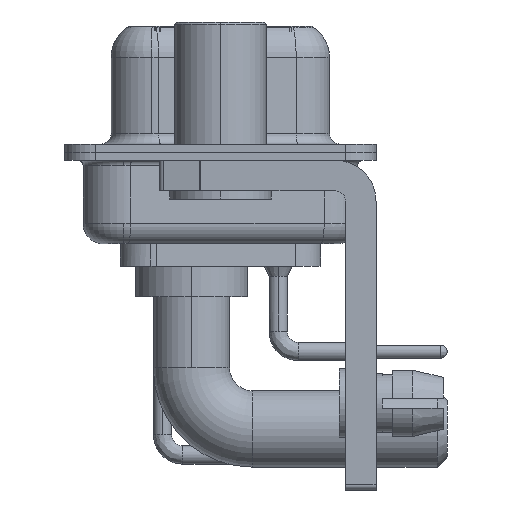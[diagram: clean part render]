
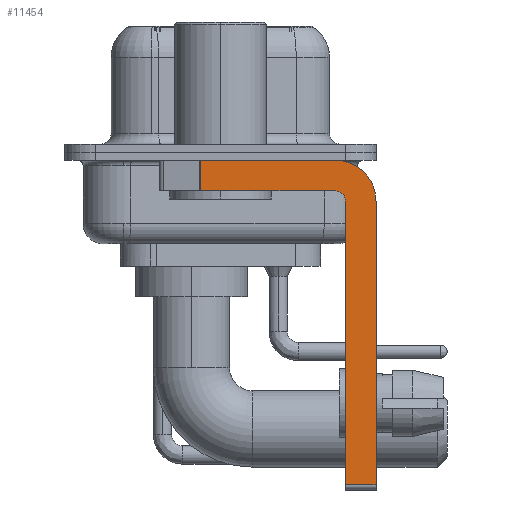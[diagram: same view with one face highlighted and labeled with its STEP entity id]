
A CAD part, left-side view. The second image highlights one B-rep face of the part: STEP entity #11454.
In plain terms, the highlighted planar face has unit normal (-1, 0, 0).
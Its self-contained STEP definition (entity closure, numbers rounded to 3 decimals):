
#1162 = DIRECTION ( 'NONE',  ( 0., 0., -1. ) ) ;
#2104 = VECTOR ( 'NONE', #4089, 1000. ) ;
#2225 = AXIS2_PLACEMENT_3D ( 'NONE', #18593, #27912, #32994 ) ;
#2735 = DIRECTION ( 'NONE',  ( 0., -1., 0. ) ) ;
#3118 = EDGE_LOOP ( 'NONE', ( #25243, #11658, #6169, #10209, #12812, #8840, #5963, #27214 ) ) ;
#4089 = DIRECTION ( 'NONE',  ( 0., 0., 1. ) ) ;
#4262 = CARTESIAN_POINT ( 'NONE',  ( -2.9, -6.15, -16.6 ) ) ;
#4948 = LINE ( 'NONE', #30495, #33307 ) ;
#5680 = CARTESIAN_POINT ( 'NONE',  ( -2.9, -6.15, -16.35 ) ) ;
#5963 = ORIENTED_EDGE ( 'NONE', *, *, #25046, .F. ) ;
#6169 = ORIENTED_EDGE ( 'NONE', *, *, #10638, .F. ) ;
#6309 = LINE ( 'NONE', #4262, #2104 ) ;
#6422 = CARTESIAN_POINT ( 'NONE',  ( -2.9, -5.65, -0.4 ) ) ;
#8209 = EDGE_CURVE ( 'NONE', #29471, #16272, #23534, .T. ) ;
#8766 = DIRECTION ( 'NONE',  ( 0., 1., 0. ) ) ;
#8840 = ORIENTED_EDGE ( 'NONE', *, *, #23420, .T. ) ;
#8956 = CARTESIAN_POINT ( 'NONE',  ( -2.9, 0.978, -1.9 ) ) ;
#9490 = CARTESIAN_POINT ( 'NONE',  ( -2.9, -5.65, -1.9 ) ) ;
#10067 = CIRCLE ( 'NONE', #13868, 2. ) ;
#10209 = ORIENTED_EDGE ( 'NONE', *, *, #29334, .F. ) ;
#10638 = EDGE_CURVE ( 'NONE', #16026, #17993, #26530, .T. ) ;
#10741 = VERTEX_POINT ( 'NONE', #32449 ) ;
#11454 = ADVANCED_FACE ( 'NONE', ( #15449 ), #25781, .F. ) ;
#11658 = ORIENTED_EDGE ( 'NONE', *, *, #25609, .T. ) ;
#12203 = DIRECTION ( 'NONE',  ( 0., 0., -1. ) ) ;
#12812 = ORIENTED_EDGE ( 'NONE', *, *, #27222, .F. ) ;
#13102 = DIRECTION ( 'NONE',  ( 1., 0., 0. ) ) ;
#13689 = CARTESIAN_POINT ( 'NONE',  ( -2.9, 0.978, -0.4 ) ) ;
#13868 = AXIS2_PLACEMENT_3D ( 'NONE', #29997, #22898, #30502 ) ;
#14150 = EDGE_CURVE ( 'NONE', #16272, #15991, #10067, .T. ) ;
#15449 = FACE_OUTER_BOUND ( 'NONE', #3118, .T. ) ;
#15776 = DIRECTION ( 'NONE',  ( 0., 0., -1. ) ) ;
#15991 = VERTEX_POINT ( 'NONE', #17605 ) ;
#16026 = VERTEX_POINT ( 'NONE', #9490 ) ;
#16272 = VERTEX_POINT ( 'NONE', #6422 ) ;
#16274 = CIRCLE ( 'NONE', #2225, 0.5 ) ;
#17193 = VERTEX_POINT ( 'NONE', #5680 ) ;
#17605 = CARTESIAN_POINT ( 'NONE',  ( -2.9, -7.65, -2.4 ) ) ;
#17993 = VERTEX_POINT ( 'NONE', #8956 ) ;
#18593 = CARTESIAN_POINT ( 'NONE',  ( -2.9, -5.65, -2.4 ) ) ;
#19361 = VECTOR ( 'NONE', #12203, 1000. ) ;
#20318 = DIRECTION ( 'NONE',  ( 0., -1., 0. ) ) ;
#20493 = CARTESIAN_POINT ( 'NONE',  ( -2.9, 3., -0.4 ) ) ;
#22898 = DIRECTION ( 'NONE',  ( 1., 0., 0. ) ) ;
#23420 = EDGE_CURVE ( 'NONE', #17193, #10741, #4948, .T. ) ;
#23534 = LINE ( 'NONE', #20493, #24619 ) ;
#24166 = CARTESIAN_POINT ( 'NONE',  ( -2.9, -5.65, -1.9 ) ) ;
#24619 = VECTOR ( 'NONE', #20318, 1000. ) ;
#24796 = VECTOR ( 'NONE', #1162, 1000. ) ;
#25046 = EDGE_CURVE ( 'NONE', #15991, #10741, #28970, .T. ) ;
#25243 = ORIENTED_EDGE ( 'NONE', *, *, #8209, .F. ) ;
#25609 = EDGE_CURVE ( 'NONE', #29471, #17993, #29602, .T. ) ;
#25781 = PLANE ( 'NONE',  #31094 ) ;
#26530 = LINE ( 'NONE', #24166, #31755 ) ;
#27214 = ORIENTED_EDGE ( 'NONE', *, *, #14150, .F. ) ;
#27222 = EDGE_CURVE ( 'NONE', #17193, #33394, #6309, .T. ) ;
#27595 = CARTESIAN_POINT ( 'NONE',  ( -2.9, -7.65, -2.4 ) ) ;
#27724 = CARTESIAN_POINT ( 'NONE',  ( -2.9, 0.978, -1.9 ) ) ;
#27912 = DIRECTION ( 'NONE',  ( -1., 0., 0. ) ) ;
#28495 = CARTESIAN_POINT ( 'NONE',  ( -2.9, -5.65, -2.4 ) ) ;
#28970 = LINE ( 'NONE', #27595, #19361 ) ;
#29334 = EDGE_CURVE ( 'NONE', #33394, #16026, #16274, .T. ) ;
#29471 = VERTEX_POINT ( 'NONE', #13689 ) ;
#29602 = LINE ( 'NONE', #27724, #24796 ) ;
#29997 = CARTESIAN_POINT ( 'NONE',  ( -2.9, -5.65, -2.4 ) ) ;
#30495 = CARTESIAN_POINT ( 'NONE',  ( -2.9, -5.65, -16.35 ) ) ;
#30502 = DIRECTION ( 'NONE',  ( 0., 0., -1. ) ) ;
#31094 = AXIS2_PLACEMENT_3D ( 'NONE', #28495, #13102, #15776 ) ;
#31755 = VECTOR ( 'NONE', #8766, 1000. ) ;
#32351 = CARTESIAN_POINT ( 'NONE',  ( -2.9, -6.15, -2.4 ) ) ;
#32449 = CARTESIAN_POINT ( 'NONE',  ( -2.9, -7.65, -16.35 ) ) ;
#32994 = DIRECTION ( 'NONE',  ( 0., 0., 1. ) ) ;
#33307 = VECTOR ( 'NONE', #2735, 1000. ) ;
#33394 = VERTEX_POINT ( 'NONE', #32351 ) ;
